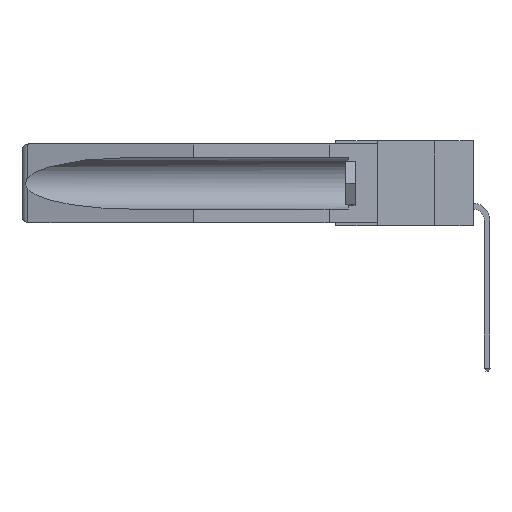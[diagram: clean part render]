
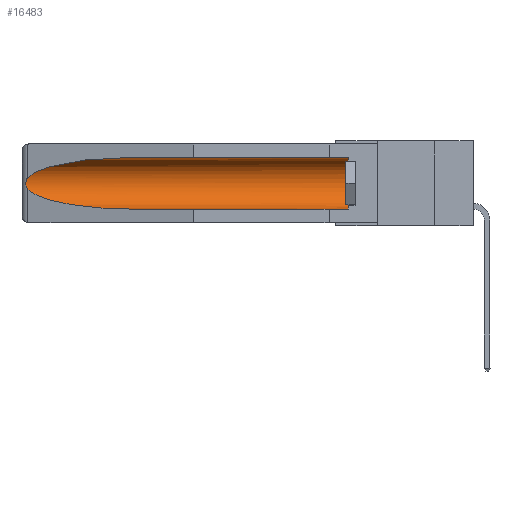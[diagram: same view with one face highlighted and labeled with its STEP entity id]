
A CAD part, left-side view. The second image highlights one B-rep face of the part: STEP entity #16483.
In plain terms, the highlighted cylindrical face has radius 2.857 mm (diameter 5.715 mm), a partial arc.
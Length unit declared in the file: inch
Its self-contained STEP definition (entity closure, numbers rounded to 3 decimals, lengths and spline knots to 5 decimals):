
#405 = ORIENTED_EDGE ( 'NONE', *, *, #8546, .T. ) ;
#571 = VERTEX_POINT ( 'NONE', #7845 ) ;
#725 = DIRECTION ( 'NONE',  ( 0., 1., 0. ) ) ;
#810 = VERTEX_POINT ( 'NONE', #17636 ) ;
#1124 = VECTOR ( 'NONE', #725, 39.37008 ) ;
#1140 = EDGE_CURVE ( 'NONE', #15303, #571, #6581, .T. ) ;
#1473 = EDGE_LOOP ( 'NONE', ( #9050, #405, #13958, #7335, #12916, #16269 ) ) ;
#1565 = CIRCLE ( 'NONE', #16827, 0.1125 ) ;
#1774 = CARTESIAN_POINT ( 'NONE',  ( 0.26537, 1.52718, -0.14972 ) ) ;
#2193 = B_SPLINE_CURVE_WITH_KNOTS ( 'NONE', 3,
 ( #9345, #8029, #2445, #6706, #13607, #4076, #5325, #17670, #13718, #12077 ),
 .UNSPECIFIED., .F., .F.,
 ( 4, 2, 2, 2, 4 ),
 ( 0., 0.00029, 0.00058, 0.00087, 0.00117 ),
 .UNSPECIFIED. ) ;
#2445 = CARTESIAN_POINT ( 'NONE',  ( 0.26654, 1.53092, -0.15636 ) ) ;
#2634 = AXIS2_PLACEMENT_3D ( 'NONE', #7384, #4830, #14489 ) ;
#3249 = DIRECTION ( 'NONE',  ( 0., -1., 0. ) ) ;
#3313 = CARTESIAN_POINT ( 'NONE',  ( 0.155, 1.07973, -0.284 ) ) ;
#3506 = CARTESIAN_POINT ( 'NONE',  ( 0.26537, 1.52718, -0.19328 ) ) ;
#3752 = EDGE_CURVE ( 'NONE', #15303, #13500, #1565, .T. ) ;
#4013 = CARTESIAN_POINT ( 'NONE',  ( 0.155, 1.07973, -0.059 ) ) ;
#4017 = CARTESIAN_POINT ( 'NONE',  ( 0.155, -0.30754, -0.284 ) ) ;
#4076 = CARTESIAN_POINT ( 'NONE',  ( 0.2675, 1.53308, -0.17534 ) ) ;
#4081 =( BOUNDED_CURVE ( )  B_SPLINE_CURVE ( 3, ( #3506, #11494, #14306, #3313 ),
 .UNSPECIFIED., .F., .F. ) 
 B_SPLINE_CURVE_WITH_KNOTS ( ( 4, 4 ),
 ( 0.1948, 1.5708 ),
 .UNSPECIFIED. ) 
 CURVE ( )  GEOMETRIC_REPRESENTATION_ITEM ( )  RATIONAL_B_SPLINE_CURVE ( ( 1., 0.848, 0.848, 1. ) ) 
 REPRESENTATION_ITEM ( '' )  );
#4830 = DIRECTION ( 'NONE',  ( 0., 1., 0. ) ) ;
#5325 = CARTESIAN_POINT ( 'NONE',  ( 0.2673, 1.53269, -0.17917 ) ) ;
#5748 = CARTESIAN_POINT ( 'NONE',  ( 0.155, 1.07973, -0.059 ) ) ;
#6581 = LINE ( 'NONE', #4017, #17184 ) ;
#6706 = CARTESIAN_POINT ( 'NONE',  ( 0.2673, 1.5327, -0.16383 ) ) ;
#7149 = LINE ( 'NONE', #17275, #1124 ) ;
#7335 = ORIENTED_EDGE ( 'NONE', *, *, #1140, .F. ) ;
#7384 = CARTESIAN_POINT ( 'NONE',  ( 0.155, -0.30754, -0.1715 ) ) ;
#7845 = CARTESIAN_POINT ( 'NONE',  ( 0.155, 1.07973, -0.284 ) ) ;
#8029 = CARTESIAN_POINT ( 'NONE',  ( 0.26597, 1.52961, -0.15275 ) ) ;
#8546 = EDGE_CURVE ( 'NONE', #9459, #810, #2193, .T. ) ;
#9050 = ORIENTED_EDGE ( 'NONE', *, *, #12873, .T. ) ;
#9345 = CARTESIAN_POINT ( 'NONE',  ( 0.26537, 1.52718, -0.14972 ) ) ;
#9398 = CARTESIAN_POINT ( 'NONE',  ( 0.155, 0.126, -0.059 ) ) ;
#9459 = VERTEX_POINT ( 'NONE', #16726 ) ;
#10012 = CARTESIAN_POINT ( 'NONE',  ( 0.21114, 1.30732, -0.059 ) ) ;
#10586 = VERTEX_POINT ( 'NONE', #4013 ) ;
#10710 = CYLINDRICAL_SURFACE ( 'NONE', #2634, 0.1125 ) ;
#11492 = CARTESIAN_POINT ( 'NONE',  ( 0.155, 0.126, -0.1715 ) ) ;
#11494 = CARTESIAN_POINT ( 'NONE',  ( 0.25451, 1.48313, -0.24835 ) ) ;
#12077 = CARTESIAN_POINT ( 'NONE',  ( 0.26537, 1.52718, -0.19328 ) ) ;
#12543 = EDGE_CURVE ( 'NONE', #13500, #10586, #7149, .T. ) ;
#12873 = EDGE_CURVE ( 'NONE', #10586, #9459, #13698, .T. ) ;
#12888 = DIRECTION ( 'NONE',  ( 0., 0., 1. ) ) ;
#12916 = ORIENTED_EDGE ( 'NONE', *, *, #3752, .T. ) ;
#13500 = VERTEX_POINT ( 'NONE', #9398 ) ;
#13607 = CARTESIAN_POINT ( 'NONE',  ( 0.2675, 1.53308, -0.16763 ) ) ;
#13698 =( BOUNDED_CURVE ( )  B_SPLINE_CURVE ( 3, ( #5748, #10012, #16986, #1774 ),
 .UNSPECIFIED., .F., .F. ) 
 B_SPLINE_CURVE_WITH_KNOTS ( ( 4, 4 ),
 ( 4.71239, 6.08839 ),
 .UNSPECIFIED. ) 
 CURVE ( )  GEOMETRIC_REPRESENTATION_ITEM ( )  RATIONAL_B_SPLINE_CURVE ( ( 1., 0.848, 0.848, 1. ) ) 
 REPRESENTATION_ITEM ( '' )  );
#13718 = CARTESIAN_POINT ( 'NONE',  ( 0.26597, 1.5296, -0.19026 ) ) ;
#13958 = ORIENTED_EDGE ( 'NONE', *, *, #14752, .T. ) ;
#14306 = CARTESIAN_POINT ( 'NONE',  ( 0.21114, 1.30732, -0.284 ) ) ;
#14489 = DIRECTION ( 'NONE',  ( 0., 0., 1. ) ) ;
#14752 = EDGE_CURVE ( 'NONE', #810, #571, #4081, .T. ) ;
#15303 = VERTEX_POINT ( 'NONE', #16508 ) ;
#16269 = ORIENTED_EDGE ( 'NONE', *, *, #12543, .T. ) ;
#16276 = DIRECTION ( 'NONE',  ( 0., 1., 0. ) ) ;
#16483 = ADVANCED_FACE ( 'NONE', ( #17664 ), #10710, .F. ) ;
#16508 = CARTESIAN_POINT ( 'NONE',  ( 0.155, 0.126, -0.284 ) ) ;
#16726 = CARTESIAN_POINT ( 'NONE',  ( 0.26537, 1.52718, -0.14972 ) ) ;
#16827 = AXIS2_PLACEMENT_3D ( 'NONE', #11492, #3249, #12888 ) ;
#16986 = CARTESIAN_POINT ( 'NONE',  ( 0.25451, 1.48313, -0.09465 ) ) ;
#17184 = VECTOR ( 'NONE', #16276, 39.37008 ) ;
#17275 = CARTESIAN_POINT ( 'NONE',  ( 0.155, -0.30754, -0.059 ) ) ;
#17636 = CARTESIAN_POINT ( 'NONE',  ( 0.26537, 1.52718, -0.19328 ) ) ;
#17664 = FACE_OUTER_BOUND ( 'NONE', #1473, .T. ) ;
#17670 = CARTESIAN_POINT ( 'NONE',  ( 0.26655, 1.53094, -0.18657 ) ) ;
